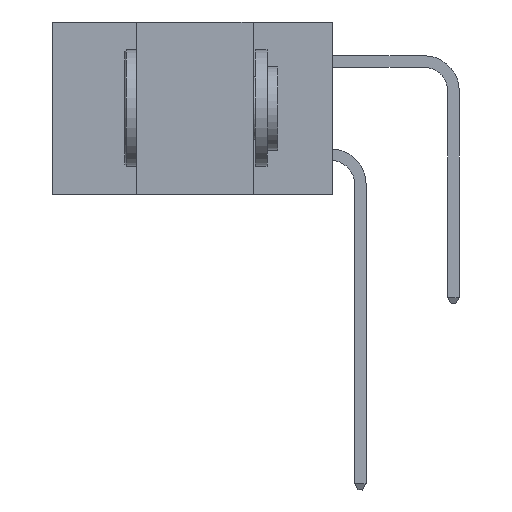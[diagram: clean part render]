
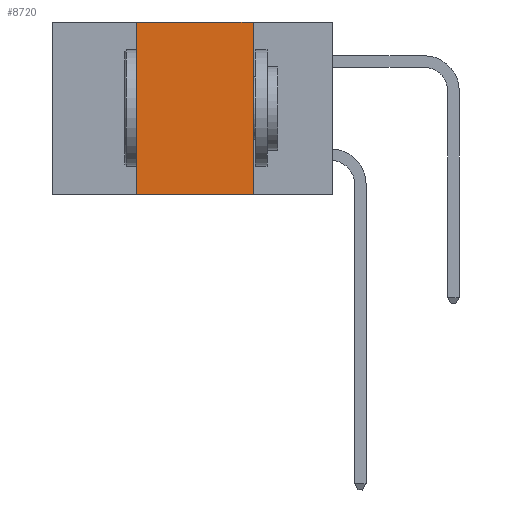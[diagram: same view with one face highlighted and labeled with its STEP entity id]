
A CAD part, left-side view. The second image highlights one B-rep face of the part: STEP entity #8720.
In plain terms, the highlighted planar face has unit normal (-1, 0, 0).
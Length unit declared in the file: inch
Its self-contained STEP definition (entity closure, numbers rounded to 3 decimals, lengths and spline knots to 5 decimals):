
#270 = PLANE ( 'NONE',  #17660 ) ;
#1289 = DIRECTION ( 'NONE',  ( 0., 0., -1. ) ) ;
#1792 = DIRECTION ( 'NONE',  ( 0., 0., -1. ) ) ;
#5153 = VECTOR ( 'NONE', #1289, 39.37008 ) ;
#5308 = LINE ( 'NONE', #12248, #12847 ) ;
#5778 = LINE ( 'NONE', #13007, #5153 ) ;
#5780 = VERTEX_POINT ( 'NONE', #18146 ) ;
#6089 = CARTESIAN_POINT ( 'NONE',  ( 0., 0.6, 0. ) ) ;
#6270 = CARTESIAN_POINT ( 'NONE',  ( 0., 0.42, -0.37 ) ) ;
#6894 = LINE ( 'NONE', #11210, #11449 ) ;
#6950 = DIRECTION ( 'NONE',  ( 0., 0., 1. ) ) ;
#7030 = VERTEX_POINT ( 'NONE', #16426 ) ;
#7124 = ORIENTED_EDGE ( 'NONE', *, *, #14301, .F. ) ;
#7477 = FACE_OUTER_BOUND ( 'NONE', #9898, .T. ) ;
#7484 = EDGE_CURVE ( 'NONE', #16694, #5780, #5308, .T. ) ;
#8144 = CARTESIAN_POINT ( 'NONE',  ( 0., 0.42, -0.37 ) ) ;
#8374 = ORIENTED_EDGE ( 'NONE', *, *, #12931, .F. ) ;
#8720 = ADVANCED_FACE ( 'NONE', ( #7477 ), #270, .F. ) ;
#9043 = VERTEX_POINT ( 'NONE', #16660 ) ;
#9202 = ORIENTED_EDGE ( 'NONE', *, *, #7484, .T. ) ;
#9890 = DIRECTION ( 'NONE',  ( 0., -1., 0. ) ) ;
#9898 = EDGE_LOOP ( 'NONE', ( #8374, #12679, #7124, #9202 ) ) ;
#11210 = CARTESIAN_POINT ( 'NONE',  ( 0., 0.6, 0. ) ) ;
#11239 = EDGE_CURVE ( 'NONE', #7030, #9043, #6894, .T. ) ;
#11449 = VECTOR ( 'NONE', #9890, 39.37008 ) ;
#11795 = DIRECTION ( 'NONE',  ( 1., 0., 0. ) ) ;
#12248 = CARTESIAN_POINT ( 'NONE',  ( 0., 0.6, -0.37 ) ) ;
#12337 = DIRECTION ( 'NONE',  ( 0., -1., 0. ) ) ;
#12679 = ORIENTED_EDGE ( 'NONE', *, *, #11239, .F. ) ;
#12847 = VECTOR ( 'NONE', #12337, 39.37008 ) ;
#12931 = EDGE_CURVE ( 'NONE', #9043, #5780, #5778, .T. ) ;
#13007 = CARTESIAN_POINT ( 'NONE',  ( 0., 0.17, -0.37 ) ) ;
#13964 = LINE ( 'NONE', #8144, #14266 ) ;
#14266 = VECTOR ( 'NONE', #6950, 39.37008 ) ;
#14301 = EDGE_CURVE ( 'NONE', #16694, #7030, #13964, .T. ) ;
#16426 = CARTESIAN_POINT ( 'NONE',  ( 0., 0.42, 0. ) ) ;
#16660 = CARTESIAN_POINT ( 'NONE',  ( 0., 0.17, 0. ) ) ;
#16694 = VERTEX_POINT ( 'NONE', #6270 ) ;
#17660 = AXIS2_PLACEMENT_3D ( 'NONE', #6089, #11795, #1792 ) ;
#18146 = CARTESIAN_POINT ( 'NONE',  ( 0., 0.17, -0.37 ) ) ;
